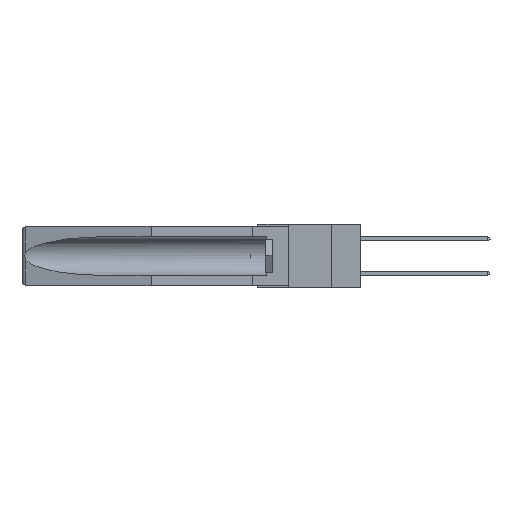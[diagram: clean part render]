
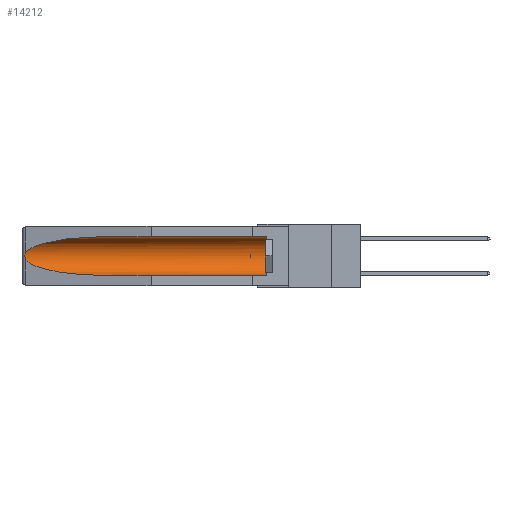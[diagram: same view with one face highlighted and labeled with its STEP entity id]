
A CAD part, left-side view. The second image highlights one B-rep face of the part: STEP entity #14212.
In plain terms, the highlighted cylindrical face has radius 2.857 mm (diameter 5.715 mm), a partial arc.
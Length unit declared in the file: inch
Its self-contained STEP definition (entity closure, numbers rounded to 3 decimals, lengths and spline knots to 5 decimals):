
#69 = CARTESIAN_POINT ( 'NONE',  ( 0.26654, 1.53092, -0.15636 ) ) ;
#375 = CARTESIAN_POINT ( 'NONE',  ( 0.155, -0.30754, -0.059 ) ) ;
#399 = EDGE_CURVE ( 'NONE', #22782, #28002, #12625, .T. ) ;
#1203 = DIRECTION ( 'NONE',  ( 0., 1., 0. ) ) ;
#1374 = CARTESIAN_POINT ( 'NONE',  ( 0.21114, 1.30732, -0.059 ) ) ;
#1597 = ORIENTED_EDGE ( 'NONE', *, *, #34407, .T. ) ;
#1888 = CARTESIAN_POINT ( 'NONE',  ( 0.26537, 1.52718, -0.14972 ) ) ;
#2965 = EDGE_CURVE ( 'NONE', #30764, #22782, #13079, .T. ) ;
#3045 = CARTESIAN_POINT ( 'NONE',  ( 0.155, 0.126, -0.1715 ) ) ;
#3848 = ORIENTED_EDGE ( 'NONE', *, *, #27419, .F. ) ;
#7332 = EDGE_CURVE ( 'NONE', #28189, #15272, #29196, .T. ) ;
#7472 = DIRECTION ( 'NONE',  ( 0., 1., 0. ) ) ;
#8267 = CARTESIAN_POINT ( 'NONE',  ( 0.26655, 1.53094, -0.18657 ) ) ;
#10626 = VERTEX_POINT ( 'NONE', #11942 ) ;
#11942 = CARTESIAN_POINT ( 'NONE',  ( 0.155, 1.07973, -0.059 ) ) ;
#11989 = CARTESIAN_POINT ( 'NONE',  ( 0.25451, 1.48313, -0.09465 ) ) ;
#12015 = CARTESIAN_POINT ( 'NONE',  ( 0.155, 1.07973, -0.284 ) ) ;
#12625 =( BOUNDED_CURVE ( )  B_SPLINE_CURVE ( 3, ( #24394, #29958, #27276, #21378 ),
 .UNSPECIFIED., .F., .T. ) 
 B_SPLINE_CURVE_WITH_KNOTS ( ( 4, 4 ),
 ( 0.1948, 1.5708 ),
 .UNSPECIFIED. ) 
 CURVE ( )  GEOMETRIC_REPRESENTATION_ITEM ( )  RATIONAL_B_SPLINE_CURVE ( ( 1., 0.848, 0.848, 1. ) ) 
 REPRESENTATION_ITEM ( '' )  );
#13079 = B_SPLINE_CURVE_WITH_KNOTS ( 'NONE', 3,
 ( #27602, #22182, #69, #13694, #30649, #33561, #19477, #8267, #27491, #16480 ),
 .UNSPECIFIED., .F., .F.,
 ( 4, 2, 2, 2, 4 ),
 ( 0., 0.00029, 0.00058, 0.00087, 0.00117 ),
 .UNSPECIFIED. ) ;
#13694 = CARTESIAN_POINT ( 'NONE',  ( 0.2673, 1.5327, -0.16383 ) ) ;
#14133 = DIRECTION ( 'NONE',  ( 0., -1., 0. ) ) ;
#14212 = ADVANCED_FACE ( 'NONE', ( #22258 ), #34397, .F. ) ;
#15272 = VERTEX_POINT ( 'NONE', #28920 ) ;
#16381 = ORIENTED_EDGE ( 'NONE', *, *, #2965, .T. ) ;
#16480 = CARTESIAN_POINT ( 'NONE',  ( 0.26537, 1.52718, -0.19328 ) ) ;
#16802 = EDGE_LOOP ( 'NONE', ( #1597, #16381, #27034, #3848, #30453, #29268 ) ) ;
#16911 = AXIS2_PLACEMENT_3D ( 'NONE', #29175, #21074, #31848 ) ;
#18097 = CARTESIAN_POINT ( 'NONE',  ( 0.155, -0.30754, -0.284 ) ) ;
#19477 = CARTESIAN_POINT ( 'NONE',  ( 0.2673, 1.53269, -0.17917 ) ) ;
#21074 = DIRECTION ( 'NONE',  ( 0., 1., 0. ) ) ;
#21378 = CARTESIAN_POINT ( 'NONE',  ( 0.155, 1.07973, -0.284 ) ) ;
#22179 = AXIS2_PLACEMENT_3D ( 'NONE', #3045, #14133, #33652 ) ;
#22182 = CARTESIAN_POINT ( 'NONE',  ( 0.26597, 1.52961, -0.15275 ) ) ;
#22258 = FACE_OUTER_BOUND ( 'NONE', #16802, .T. ) ;
#22782 = VERTEX_POINT ( 'NONE', #33457 ) ;
#23590 = VECTOR ( 'NONE', #7472, 39.37008 ) ;
#24394 = CARTESIAN_POINT ( 'NONE',  ( 0.26537, 1.52718, -0.19328 ) ) ;
#26195 = VECTOR ( 'NONE', #1203, 39.37008 ) ;
#27034 = ORIENTED_EDGE ( 'NONE', *, *, #399, .T. ) ;
#27176 = EDGE_CURVE ( 'NONE', #15272, #10626, #34893, .T. ) ;
#27276 = CARTESIAN_POINT ( 'NONE',  ( 0.21114, 1.30732, -0.284 ) ) ;
#27419 = EDGE_CURVE ( 'NONE', #28189, #28002, #33577, .T. ) ;
#27491 = CARTESIAN_POINT ( 'NONE',  ( 0.26597, 1.5296, -0.19026 ) ) ;
#27602 = CARTESIAN_POINT ( 'NONE',  ( 0.26537, 1.52718, -0.14972 ) ) ;
#28002 = VERTEX_POINT ( 'NONE', #12015 ) ;
#28189 = VERTEX_POINT ( 'NONE', #33199 ) ;
#28556 = CARTESIAN_POINT ( 'NONE',  ( 0.155, 1.07973, -0.059 ) ) ;
#28674 = CARTESIAN_POINT ( 'NONE',  ( 0.26537, 1.52718, -0.14972 ) ) ;
#28920 = CARTESIAN_POINT ( 'NONE',  ( 0.155, 0.126, -0.059 ) ) ;
#29175 = CARTESIAN_POINT ( 'NONE',  ( 0.155, -0.30754, -0.1715 ) ) ;
#29196 = CIRCLE ( 'NONE', #22179, 0.1125 ) ;
#29268 = ORIENTED_EDGE ( 'NONE', *, *, #27176, .T. ) ;
#29958 = CARTESIAN_POINT ( 'NONE',  ( 0.25451, 1.48313, -0.24835 ) ) ;
#30453 = ORIENTED_EDGE ( 'NONE', *, *, #7332, .T. ) ;
#30649 = CARTESIAN_POINT ( 'NONE',  ( 0.2675, 1.53308, -0.16763 ) ) ;
#30764 = VERTEX_POINT ( 'NONE', #1888 ) ;
#31848 = DIRECTION ( 'NONE',  ( 0., 0., 1. ) ) ;
#32618 =( BOUNDED_CURVE ( )  B_SPLINE_CURVE ( 3, ( #28556, #1374, #11989, #28674 ),
 .UNSPECIFIED., .F., .F. ) 
 B_SPLINE_CURVE_WITH_KNOTS ( ( 4, 4 ),
 ( 4.71239, 6.08839 ),
 .UNSPECIFIED. ) 
 CURVE ( )  GEOMETRIC_REPRESENTATION_ITEM ( )  RATIONAL_B_SPLINE_CURVE ( ( 1., 0.848, 0.848, 1. ) ) 
 REPRESENTATION_ITEM ( '' )  );
#33199 = CARTESIAN_POINT ( 'NONE',  ( 0.155, 0.126, -0.284 ) ) ;
#33457 = CARTESIAN_POINT ( 'NONE',  ( 0.26537, 1.52718, -0.19328 ) ) ;
#33561 = CARTESIAN_POINT ( 'NONE',  ( 0.2675, 1.53308, -0.17534 ) ) ;
#33577 = LINE ( 'NONE', #18097, #23590 ) ;
#33652 = DIRECTION ( 'NONE',  ( 0., 0., 1. ) ) ;
#34397 = CYLINDRICAL_SURFACE ( 'NONE', #16911, 0.1125 ) ;
#34407 = EDGE_CURVE ( 'NONE', #10626, #30764, #32618, .T. ) ;
#34893 = LINE ( 'NONE', #375, #26195 ) ;
